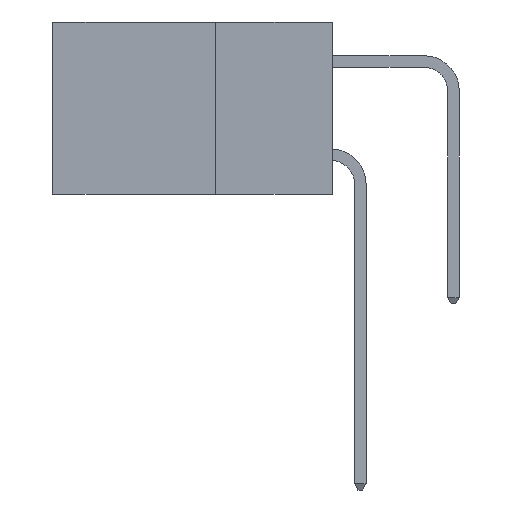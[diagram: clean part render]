
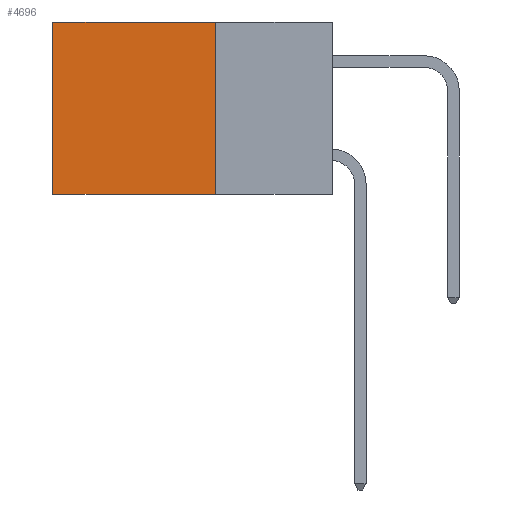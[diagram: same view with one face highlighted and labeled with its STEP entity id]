
A CAD part, left-side view. The second image highlights one B-rep face of the part: STEP entity #4696.
In plain terms, the highlighted planar face has unit normal (-1, 0, 0).
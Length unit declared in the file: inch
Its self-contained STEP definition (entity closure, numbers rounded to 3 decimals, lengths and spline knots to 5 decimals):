
#917 = ORIENTED_EDGE ( 'NONE', *, *, #10029, .F. ) ;
#1627 = VERTEX_POINT ( 'NONE', #7256 ) ;
#1726 = DIRECTION ( 'NONE',  ( 0., 0., -1. ) ) ;
#1971 = VECTOR ( 'NONE', #6747, 39.37008 ) ;
#2128 = ORIENTED_EDGE ( 'NONE', *, *, #13716, .T. ) ;
#2489 = DIRECTION ( 'NONE',  ( 0., 0., -1. ) ) ;
#2490 = FACE_OUTER_BOUND ( 'NONE', #17612, .T. ) ;
#2572 = DIRECTION ( 'NONE',  ( 1., 0., 0. ) ) ;
#2678 = CARTESIAN_POINT ( 'NONE',  ( 0.2615, 0.25, -0.37 ) ) ;
#2732 = PLANE ( 'NONE',  #11428 ) ;
#3420 = VERTEX_POINT ( 'NONE', #6974 ) ;
#3592 = LINE ( 'NONE', #12145, #7140 ) ;
#4696 = ADVANCED_FACE ( 'NONE', ( #2490 ), #2732, .F. ) ;
#5193 = LINE ( 'NONE', #9118, #13056 ) ;
#5660 = EDGE_CURVE ( 'NONE', #3420, #1627, #17723, .T. ) ;
#5824 = DIRECTION ( 'NONE',  ( 0., 1., 0. ) ) ;
#5844 = CARTESIAN_POINT ( 'NONE',  ( 0.2615, 0.25, -0.37 ) ) ;
#5999 = ORIENTED_EDGE ( 'NONE', *, *, #7378, .F. ) ;
#6150 = CARTESIAN_POINT ( 'NONE',  ( 0.2615, 0.25, -0.37 ) ) ;
#6273 = VERTEX_POINT ( 'NONE', #5844 ) ;
#6436 = VECTOR ( 'NONE', #5824, 39.37008 ) ;
#6747 = DIRECTION ( 'NONE',  ( 0., 1., 0. ) ) ;
#6756 = CARTESIAN_POINT ( 'NONE',  ( 0.2615, 0.6, -0.37 ) ) ;
#6974 = CARTESIAN_POINT ( 'NONE',  ( 0.2615, 0.25, 0. ) ) ;
#7140 = VECTOR ( 'NONE', #1726, 39.37008 ) ;
#7256 = CARTESIAN_POINT ( 'NONE',  ( 0.2615, 0.6, 0. ) ) ;
#7378 = EDGE_CURVE ( 'NONE', #6273, #12680, #14257, .T. ) ;
#7682 = CARTESIAN_POINT ( 'NONE',  ( 0.2615, 0.25, 0. ) ) ;
#9118 = CARTESIAN_POINT ( 'NONE',  ( 0.2615, 0.25, -0.37 ) ) ;
#10029 = EDGE_CURVE ( 'NONE', #3420, #6273, #5193, .T. ) ;
#10584 = DIRECTION ( 'NONE',  ( 0., 0., -1. ) ) ;
#11428 = AXIS2_PLACEMENT_3D ( 'NONE', #2678, #2572, #2489 ) ;
#12145 = CARTESIAN_POINT ( 'NONE',  ( 0.2615, 0.6, -0.37 ) ) ;
#12680 = VERTEX_POINT ( 'NONE', #6756 ) ;
#13056 = VECTOR ( 'NONE', #10584, 39.37008 ) ;
#13716 = EDGE_CURVE ( 'NONE', #1627, #12680, #3592, .T. ) ;
#14257 = LINE ( 'NONE', #6150, #6436 ) ;
#17612 = EDGE_LOOP ( 'NONE', ( #2128, #5999, #917, #18557 ) ) ;
#17723 = LINE ( 'NONE', #7682, #1971 ) ;
#18557 = ORIENTED_EDGE ( 'NONE', *, *, #5660, .T. ) ;
